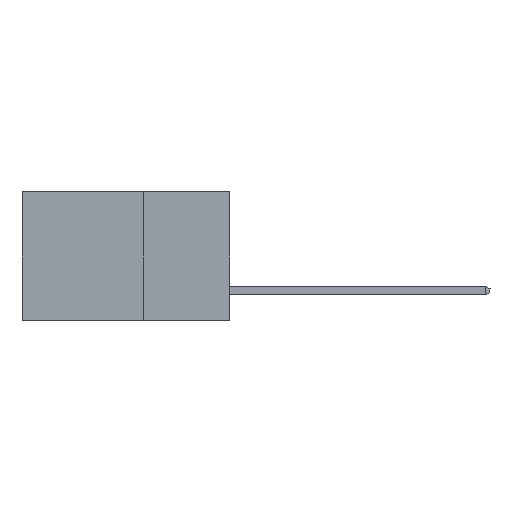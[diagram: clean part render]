
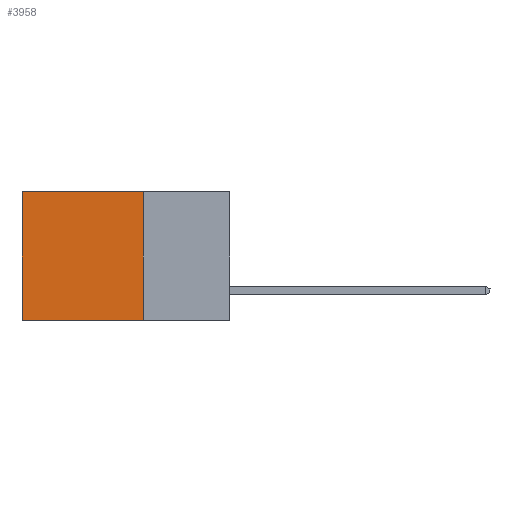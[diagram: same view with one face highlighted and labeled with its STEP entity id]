
A CAD part, left-side view. The second image highlights one B-rep face of the part: STEP entity #3958.
In plain terms, the highlighted planar face has unit normal (-1, 0, 0).
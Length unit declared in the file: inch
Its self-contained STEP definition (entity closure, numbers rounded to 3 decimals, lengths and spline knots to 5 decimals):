
#159 = EDGE_CURVE ( 'NONE', #3037, #4436, #3677, .T. ) ;
#164 = EDGE_LOOP ( 'NONE', ( #9254, #4521, #4840, #6985 ) ) ;
#201 = CARTESIAN_POINT ( 'NONE',  ( 0.2615, 0.25, -0.37 ) ) ;
#263 = LINE ( 'NONE', #2218, #11337 ) ;
#1077 = LINE ( 'NONE', #6893, #3943 ) ;
#1110 = CARTESIAN_POINT ( 'NONE',  ( 0.2615, 0.6, -0.37 ) ) ;
#1429 = VERTEX_POINT ( 'NONE', #1110 ) ;
#1675 = LINE ( 'NONE', #2591, #6531 ) ;
#2218 = CARTESIAN_POINT ( 'NONE',  ( 0.2615, 0.6, -0.37 ) ) ;
#2525 = AXIS2_PLACEMENT_3D ( 'NONE', #3488, #11674, #5641 ) ;
#2591 = CARTESIAN_POINT ( 'NONE',  ( 0.2615, 0.25, -0.37 ) ) ;
#3037 = VERTEX_POINT ( 'NONE', #4374 ) ;
#3488 = CARTESIAN_POINT ( 'NONE',  ( 0.2615, 0.25, -0.37 ) ) ;
#3677 = LINE ( 'NONE', #3736, #10091 ) ;
#3701 = EDGE_CURVE ( 'NONE', #3037, #7694, #1077, .T. ) ;
#3736 = CARTESIAN_POINT ( 'NONE',  ( 0.2615, 0.25, 0. ) ) ;
#3943 = VECTOR ( 'NONE', #9980, 39.37008 ) ;
#3958 = ADVANCED_FACE ( 'NONE', ( #7680 ), #10552, .F. ) ;
#4374 = CARTESIAN_POINT ( 'NONE',  ( 0.2615, 0.25, 0. ) ) ;
#4436 = VERTEX_POINT ( 'NONE', #11510 ) ;
#4521 = ORIENTED_EDGE ( 'NONE', *, *, #8205, .F. ) ;
#4840 = ORIENTED_EDGE ( 'NONE', *, *, #3701, .F. ) ;
#5641 = DIRECTION ( 'NONE',  ( 0., 0., -1. ) ) ;
#6531 = VECTOR ( 'NONE', #9542, 39.37008 ) ;
#6893 = CARTESIAN_POINT ( 'NONE',  ( 0.2615, 0.25, -0.37 ) ) ;
#6985 = ORIENTED_EDGE ( 'NONE', *, *, #159, .T. ) ;
#7680 = FACE_OUTER_BOUND ( 'NONE', #164, .T. ) ;
#7694 = VERTEX_POINT ( 'NONE', #201 ) ;
#7711 = EDGE_CURVE ( 'NONE', #4436, #1429, #263, .T. ) ;
#8205 = EDGE_CURVE ( 'NONE', #7694, #1429, #1675, .T. ) ;
#8849 = DIRECTION ( 'NONE',  ( 0., 1., 0. ) ) ;
#9254 = ORIENTED_EDGE ( 'NONE', *, *, #7711, .T. ) ;
#9542 = DIRECTION ( 'NONE',  ( 0., 1., 0. ) ) ;
#9980 = DIRECTION ( 'NONE',  ( 0., 0., -1. ) ) ;
#10091 = VECTOR ( 'NONE', #8849, 39.37008 ) ;
#10552 = PLANE ( 'NONE',  #2525 ) ;
#11337 = VECTOR ( 'NONE', #12241, 39.37008 ) ;
#11510 = CARTESIAN_POINT ( 'NONE',  ( 0.2615, 0.6, 0. ) ) ;
#11674 = DIRECTION ( 'NONE',  ( 1., 0., 0. ) ) ;
#12241 = DIRECTION ( 'NONE',  ( 0., 0., -1. ) ) ;
